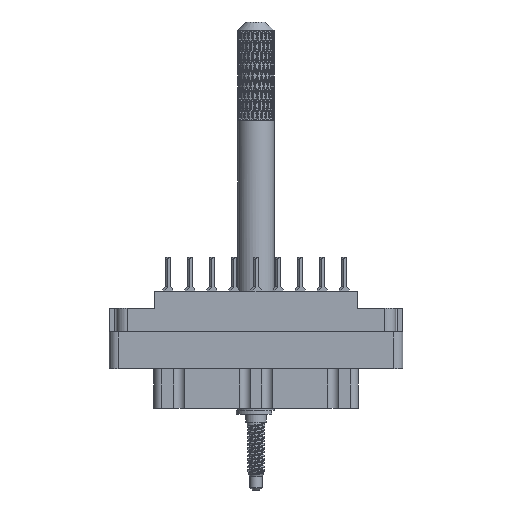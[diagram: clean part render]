
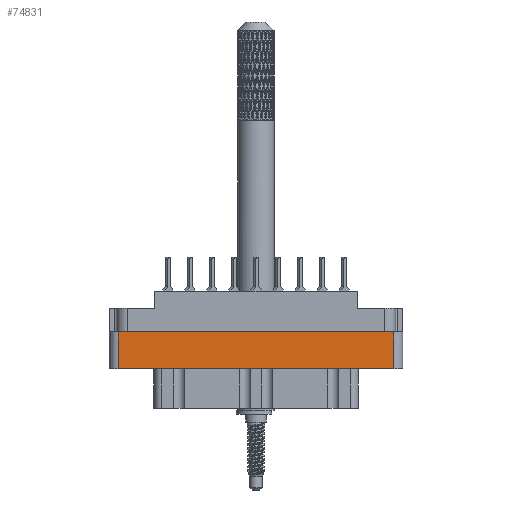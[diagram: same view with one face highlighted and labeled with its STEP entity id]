
A CAD part, front view. The second image highlights one B-rep face of the part: STEP entity #74831.
In plain terms, the highlighted planar face has unit normal (0, -1, 0).
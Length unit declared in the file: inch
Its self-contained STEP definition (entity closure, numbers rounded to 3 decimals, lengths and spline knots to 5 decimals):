
#1496 = LINE ( 'NONE', #47495, #36862 ) ;
#5619 = VERTEX_POINT ( 'NONE', #40882 ) ;
#10821 = ORIENTED_EDGE ( 'NONE', *, *, #34643, .F. ) ;
#10995 = CARTESIAN_POINT ( 'NONE',  ( 0.938, -0.438, -0.529 ) ) ;
#14908 = AXIS2_PLACEMENT_3D ( 'NONE', #99768, #29004, #60539 ) ;
#16004 = DIRECTION ( 'NONE',  ( 1., 0., 0. ) ) ;
#18046 = VECTOR ( 'NONE', #84495, 39.37008 ) ;
#18225 = LINE ( 'NONE', #72979, #83084 ) ;
#28114 = CARTESIAN_POINT ( 'NONE',  ( 0.938, -0.438, -0.529 ) ) ;
#28719 = LINE ( 'NONE', #59747, #18046 ) ;
#29004 = DIRECTION ( 'NONE',  ( 0., -1., 0. ) ) ;
#34643 = EDGE_CURVE ( 'NONE', #81641, #5619, #18225, .T. ) ;
#36763 = FACE_OUTER_BOUND ( 'NONE', #37278, .T. ) ;
#36862 = VECTOR ( 'NONE', #16004, 39.37008 ) ;
#37278 = EDGE_LOOP ( 'NONE', ( #10821, #59914, #37665, #62151 ) ) ;
#37665 = ORIENTED_EDGE ( 'NONE', *, *, #79666, .T. ) ;
#40882 = CARTESIAN_POINT ( 'NONE',  ( -0.938, -0.438, -0.277 ) ) ;
#47495 = CARTESIAN_POINT ( 'NONE',  ( -1., -0.438, -0.277 ) ) ;
#50526 = CARTESIAN_POINT ( 'NONE',  ( -0.938, -0.438, -0.529 ) ) ;
#53430 = LINE ( 'NONE', #28114, #54175 ) ;
#54175 = VECTOR ( 'NONE', #60679, 39.37008 ) ;
#59747 = CARTESIAN_POINT ( 'NONE',  ( 0.938, -0.438, -0.798 ) ) ;
#59914 = ORIENTED_EDGE ( 'NONE', *, *, #60581, .F. ) ;
#60539 = DIRECTION ( 'NONE',  ( 0., 0., -1. ) ) ;
#60581 = EDGE_CURVE ( 'NONE', #60819, #81641, #53430, .T. ) ;
#60679 = DIRECTION ( 'NONE',  ( -1., 0., 0. ) ) ;
#60819 = VERTEX_POINT ( 'NONE', #10995 ) ;
#62151 = ORIENTED_EDGE ( 'NONE', *, *, #98160, .F. ) ;
#67078 = CARTESIAN_POINT ( 'NONE',  ( 0.938, -0.438, -0.277 ) ) ;
#68283 = PLANE ( 'NONE',  #14908 ) ;
#72979 = CARTESIAN_POINT ( 'NONE',  ( -0.938, -0.438, -0.798 ) ) ;
#74831 = ADVANCED_FACE ( 'NONE', ( #36763 ), #68283, .T. ) ;
#79666 = EDGE_CURVE ( 'NONE', #60819, #82735, #28719, .T. ) ;
#81641 = VERTEX_POINT ( 'NONE', #50526 ) ;
#82735 = VERTEX_POINT ( 'NONE', #67078 ) ;
#83084 = VECTOR ( 'NONE', #95675, 39.37008 ) ;
#84495 = DIRECTION ( 'NONE',  ( 0., 0., 1. ) ) ;
#95675 = DIRECTION ( 'NONE',  ( 0., 0., 1. ) ) ;
#98160 = EDGE_CURVE ( 'NONE', #5619, #82735, #1496, .T. ) ;
#99768 = CARTESIAN_POINT ( 'NONE',  ( -0.938, -0.438, -0.798 ) ) ;
